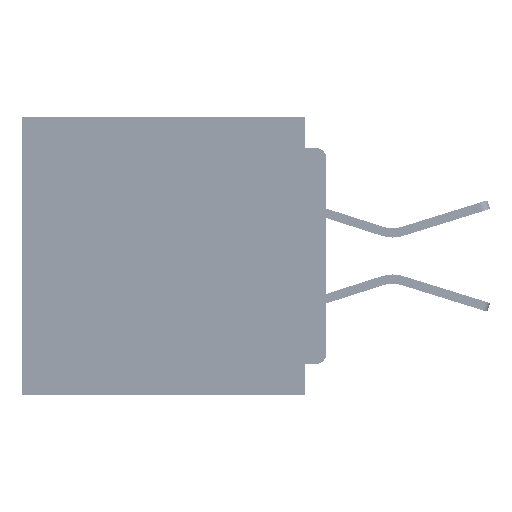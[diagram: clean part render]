
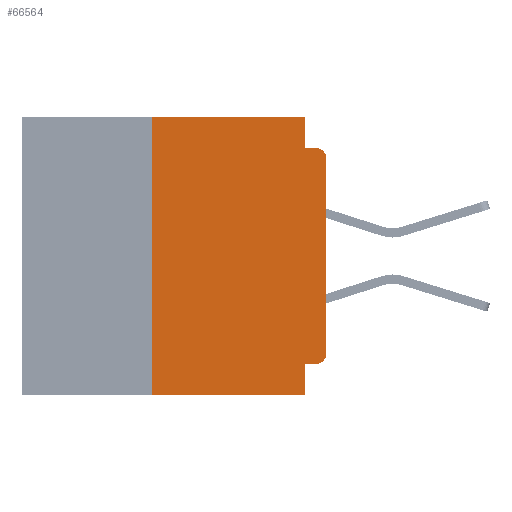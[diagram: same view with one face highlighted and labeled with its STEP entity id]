
A CAD part, left-side view. The second image highlights one B-rep face of the part: STEP entity #66564.
In plain terms, the highlighted planar face has unit normal (-1, 0, 0).
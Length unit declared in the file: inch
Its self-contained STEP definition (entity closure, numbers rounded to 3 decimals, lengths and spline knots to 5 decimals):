
#1016 = CARTESIAN_POINT ( 'NONE',  ( 0., 0.437, 0. ) ) ;
#1138 = VERTEX_POINT ( 'NONE', #12519 ) ;
#1227 = VERTEX_POINT ( 'NONE', #8409 ) ;
#1643 = EDGE_CURVE ( 'NONE', #48512, #14307, #63239, .T. ) ;
#1834 = VERTEX_POINT ( 'NONE', #66007 ) ;
#2372 = CARTESIAN_POINT ( 'NONE',  ( 0., 0., -0.34 ) ) ;
#2990 = EDGE_LOOP ( 'NONE', ( #30170, #19882, #27290, #6971, #4532, #52736, #59894, #17643, #10654, #33274 ) ) ;
#3604 = CARTESIAN_POINT ( 'NONE',  ( 0., 0.031, -0.4 ) ) ;
#3937 = EDGE_CURVE ( 'NONE', #14307, #1138, #12612, .T. ) ;
#4532 = ORIENTED_EDGE ( 'NONE', *, *, #1643, .F. ) ;
#6837 = FACE_OUTER_BOUND ( 'NONE', #2990, .T. ) ;
#6971 = ORIENTED_EDGE ( 'NONE', *, *, #3937, .F. ) ;
#7233 = CIRCLE ( 'NONE', #63488, 0.015 ) ;
#8098 = DIRECTION ( 'NONE',  ( 0., 0., -1. ) ) ;
#8409 = CARTESIAN_POINT ( 'NONE',  ( 0., 0.25, -0.4 ) ) ;
#10654 = ORIENTED_EDGE ( 'NONE', *, *, #18897, .F. ) ;
#11557 = CARTESIAN_POINT ( 'NONE',  ( 0., 0.031, -0.355 ) ) ;
#12519 = CARTESIAN_POINT ( 'NONE',  ( 0., 0.031, -0.045 ) ) ;
#12612 = LINE ( 'NONE', #16077, #66954 ) ;
#13032 = EDGE_CURVE ( 'NONE', #1227, #48512, #37228, .T. ) ;
#13820 = CARTESIAN_POINT ( 'NONE',  ( 0., 0.015, -0.34 ) ) ;
#14307 = VERTEX_POINT ( 'NONE', #34561 ) ;
#15462 = VECTOR ( 'NONE', #28598, 39.37008 ) ;
#16077 = CARTESIAN_POINT ( 'NONE',  ( 0., 0.031, 0. ) ) ;
#16592 = VECTOR ( 'NONE', #8098, 39.37008 ) ;
#17643 = ORIENTED_EDGE ( 'NONE', *, *, #63604, .F. ) ;
#18224 = CIRCLE ( 'NONE', #47250, 0.015 ) ;
#18707 = DIRECTION ( 'NONE',  ( 0., -1., 0. ) ) ;
#18897 = EDGE_CURVE ( 'NONE', #1834, #61969, #46766, .T. ) ;
#19158 = DIRECTION ( 'NONE',  ( 0., 0., -1. ) ) ;
#19882 = ORIENTED_EDGE ( 'NONE', *, *, #45245, .T. ) ;
#20587 = VERTEX_POINT ( 'NONE', #3604 ) ;
#20746 = VECTOR ( 'NONE', #18707, 39.37008 ) ;
#20972 = DIRECTION ( 'NONE',  ( 0., 0., 1. ) ) ;
#21076 = EDGE_CURVE ( 'NONE', #60914, #51907, #56274, .T. ) ;
#21392 = DIRECTION ( 'NONE',  ( 0., 0., -1. ) ) ;
#21451 = CARTESIAN_POINT ( 'NONE',  ( 0., 0.015, -0.06 ) ) ;
#23794 = CARTESIAN_POINT ( 'NONE',  ( 0., 0.437, -0.4 ) ) ;
#24313 = AXIS2_PLACEMENT_3D ( 'NONE', #46122, #67102, #35822 ) ;
#24380 = EDGE_CURVE ( 'NONE', #1138, #62737, #42005, .T. ) ;
#26808 = DIRECTION ( 'NONE',  ( 0., 0., -1. ) ) ;
#27290 = ORIENTED_EDGE ( 'NONE', *, *, #24380, .F. ) ;
#28286 = VECTOR ( 'NONE', #61516, 39.37008 ) ;
#28598 = DIRECTION ( 'NONE',  ( 0., -1., 0. ) ) ;
#29418 = VECTOR ( 'NONE', #63959, 39.37008 ) ;
#30170 = ORIENTED_EDGE ( 'NONE', *, *, #21076, .T. ) ;
#30454 = PLANE ( 'NONE',  #24313 ) ;
#33274 = ORIENTED_EDGE ( 'NONE', *, *, #56161, .T. ) ;
#34561 = CARTESIAN_POINT ( 'NONE',  ( 0., 0.031, 0. ) ) ;
#34895 = LINE ( 'NONE', #23794, #20746 ) ;
#35822 = DIRECTION ( 'NONE',  ( 0., 0., -1. ) ) ;
#37228 = LINE ( 'NONE', #47085, #63379 ) ;
#40495 = CARTESIAN_POINT ( 'NONE',  ( 0., 0., 0. ) ) ;
#42005 = LINE ( 'NONE', #60091, #15462 ) ;
#45245 = EDGE_CURVE ( 'NONE', #51907, #62737, #7233, .T. ) ;
#45966 = CARTESIAN_POINT ( 'NONE',  ( 0., 0.25, 0. ) ) ;
#46122 = CARTESIAN_POINT ( 'NONE',  ( 0., 0.437, 0. ) ) ;
#46766 = LINE ( 'NONE', #48182, #29418 ) ;
#47085 = CARTESIAN_POINT ( 'NONE',  ( 0., 0.25, -0.4 ) ) ;
#47250 = AXIS2_PLACEMENT_3D ( 'NONE', #13820, #50759, #19158 ) ;
#48182 = CARTESIAN_POINT ( 'NONE',  ( 0., 0., -0.355 ) ) ;
#48512 = VERTEX_POINT ( 'NONE', #45966 ) ;
#49317 = VECTOR ( 'NONE', #64222, 39.37008 ) ;
#50259 = EDGE_CURVE ( 'NONE', #1227, #20587, #34895, .T. ) ;
#50759 = DIRECTION ( 'NONE',  ( -1., 0., 0. ) ) ;
#51907 = VERTEX_POINT ( 'NONE', #61397 ) ;
#52736 = ORIENTED_EDGE ( 'NONE', *, *, #13032, .F. ) ;
#56161 = EDGE_CURVE ( 'NONE', #1834, #60914, #18224, .T. ) ;
#56274 = LINE ( 'NONE', #40495, #28286 ) ;
#58320 = DIRECTION ( 'NONE',  ( -1., 0., 0. ) ) ;
#58651 = LINE ( 'NONE', #65910, #16592 ) ;
#59894 = ORIENTED_EDGE ( 'NONE', *, *, #50259, .T. ) ;
#60091 = CARTESIAN_POINT ( 'NONE',  ( 0., 0., -0.045 ) ) ;
#60914 = VERTEX_POINT ( 'NONE', #2372 ) ;
#61397 = CARTESIAN_POINT ( 'NONE',  ( 0., 0., -0.06 ) ) ;
#61516 = DIRECTION ( 'NONE',  ( 0., 0., 1. ) ) ;
#61969 = VERTEX_POINT ( 'NONE', #11557 ) ;
#62737 = VERTEX_POINT ( 'NONE', #64211 ) ;
#63239 = LINE ( 'NONE', #1016, #49317 ) ;
#63379 = VECTOR ( 'NONE', #20972, 39.37008 ) ;
#63488 = AXIS2_PLACEMENT_3D ( 'NONE', #21451, #58320, #26808 ) ;
#63604 = EDGE_CURVE ( 'NONE', #61969, #20587, #58651, .T. ) ;
#63959 = DIRECTION ( 'NONE',  ( 0., 1., 0. ) ) ;
#64211 = CARTESIAN_POINT ( 'NONE',  ( 0., 0.015, -0.045 ) ) ;
#64222 = DIRECTION ( 'NONE',  ( 0., -1., 0. ) ) ;
#65910 = CARTESIAN_POINT ( 'NONE',  ( 0., 0.031, -0.4 ) ) ;
#66007 = CARTESIAN_POINT ( 'NONE',  ( 0., 0.015, -0.355 ) ) ;
#66564 = ADVANCED_FACE ( 'NONE', ( #6837 ), #30454, .F. ) ;
#66954 = VECTOR ( 'NONE', #21392, 39.37008 ) ;
#67102 = DIRECTION ( 'NONE',  ( 1., 0., 0. ) ) ;
